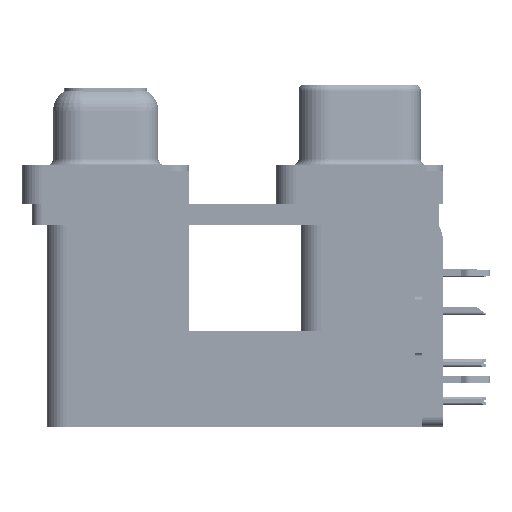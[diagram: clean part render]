
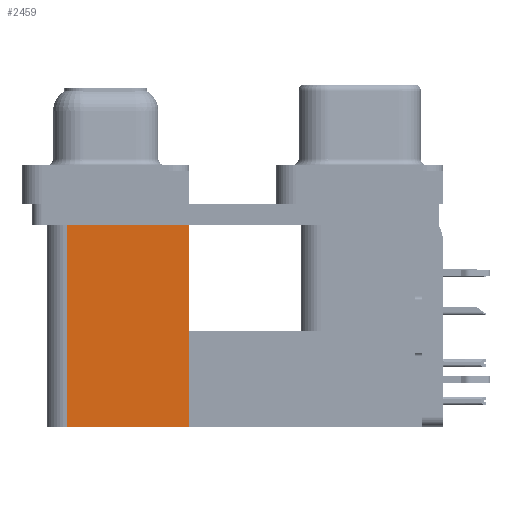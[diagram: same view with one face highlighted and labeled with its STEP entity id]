
A CAD part, left-side view. The second image highlights one B-rep face of the part: STEP entity #2459.
In plain terms, the highlighted planar face has unit normal (-1, 0, 0).
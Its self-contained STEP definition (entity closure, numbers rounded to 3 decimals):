
#59 = CARTESIAN_POINT ( 'NONE',  ( 3.79, 21.975, -19.2 ) ) ;
#288 = EDGE_LOOP ( 'NONE', ( #23980, #52219, #5818, #51550 ) ) ;
#2200 = VERTEX_POINT ( 'NONE', #3281 ) ;
#2459 = ADVANCED_FACE ( 'NONE', ( #51339 ), #20069, .F. ) ;
#3281 = CARTESIAN_POINT ( 'NONE',  ( 3.79, 12.775, -2.5 ) ) ;
#5041 = CARTESIAN_POINT ( 'NONE',  ( 3.79, 12.775, -19.2 ) ) ;
#5818 = ORIENTED_EDGE ( 'NONE', *, *, #15808, .F. ) ;
#6556 = CARTESIAN_POINT ( 'NONE',  ( 3.79, 12.775, -2.5 ) ) ;
#9904 = CARTESIAN_POINT ( 'NONE',  ( 3.79, 12.775, -19.2 ) ) ;
#10181 = LINE ( 'NONE', #5041, #46374 ) ;
#13522 = VERTEX_POINT ( 'NONE', #9904 ) ;
#15808 = EDGE_CURVE ( 'NONE', #13522, #62900, #48556, .T. ) ;
#15822 = LINE ( 'NONE', #6556, #32782 ) ;
#17273 = CARTESIAN_POINT ( 'NONE',  ( 3.79, 12.775, -19.2 ) ) ;
#19368 = CARTESIAN_POINT ( 'NONE',  ( 3.79, 21.975, -2.5 ) ) ;
#19542 = VECTOR ( 'NONE', #42358, 1000. ) ;
#20069 = PLANE ( 'NONE',  #36291 ) ;
#21535 = VERTEX_POINT ( 'NONE', #19368 ) ;
#23980 = ORIENTED_EDGE ( 'NONE', *, *, #57555, .T. ) ;
#29025 = LINE ( 'NONE', #49996, #34534 ) ;
#32782 = VECTOR ( 'NONE', #63918, 1000. ) ;
#34534 = VECTOR ( 'NONE', #56846, 1000. ) ;
#36044 = EDGE_CURVE ( 'NONE', #62900, #21535, #29025, .T. ) ;
#36178 = CARTESIAN_POINT ( 'NONE',  ( 3.79, 12.775, -19.2 ) ) ;
#36291 = AXIS2_PLACEMENT_3D ( 'NONE', #36178, #45176, #66142 ) ;
#42358 = DIRECTION ( 'NONE',  ( 0., 1., 0. ) ) ;
#45176 = DIRECTION ( 'NONE',  ( 1., 0., 0. ) ) ;
#46374 = VECTOR ( 'NONE', #51080, 1000. ) ;
#48556 = LINE ( 'NONE', #17273, #19542 ) ;
#49996 = CARTESIAN_POINT ( 'NONE',  ( 3.79, 21.975, -19.2 ) ) ;
#51080 = DIRECTION ( 'NONE',  ( 0., 0., 1. ) ) ;
#51339 = FACE_OUTER_BOUND ( 'NONE', #288, .T. ) ;
#51550 = ORIENTED_EDGE ( 'NONE', *, *, #61994, .T. ) ;
#52219 = ORIENTED_EDGE ( 'NONE', *, *, #36044, .F. ) ;
#56846 = DIRECTION ( 'NONE',  ( 0., 0., 1. ) ) ;
#57555 = EDGE_CURVE ( 'NONE', #2200, #21535, #15822, .T. ) ;
#61994 = EDGE_CURVE ( 'NONE', #13522, #2200, #10181, .T. ) ;
#62900 = VERTEX_POINT ( 'NONE', #59 ) ;
#63918 = DIRECTION ( 'NONE',  ( 0., 1., 0. ) ) ;
#66142 = DIRECTION ( 'NONE',  ( 0., 1., 0. ) ) ;
